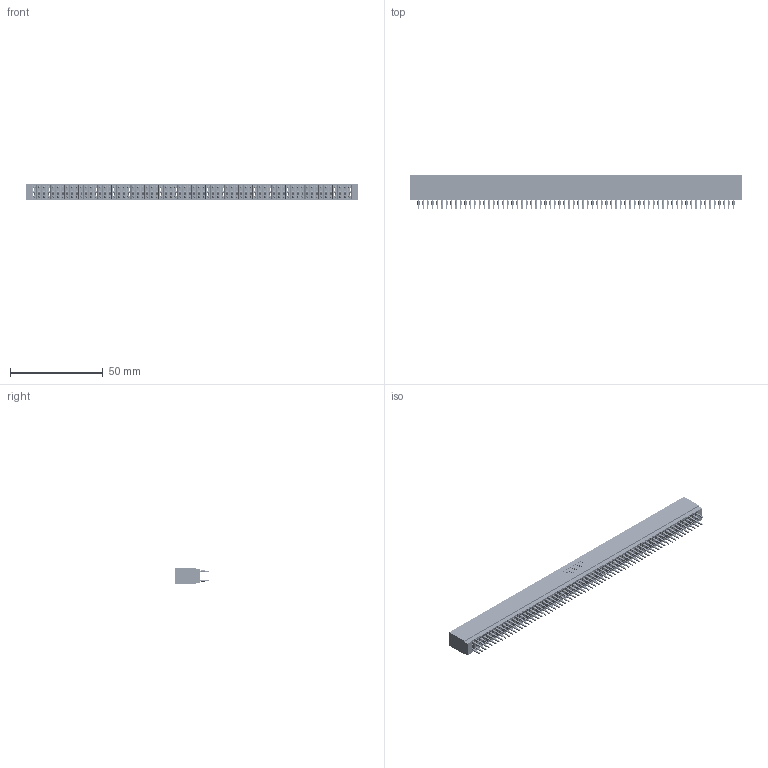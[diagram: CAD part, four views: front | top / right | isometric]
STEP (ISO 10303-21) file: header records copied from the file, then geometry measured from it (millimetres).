
FILE_DESCRIPTION (( 'STEP AP203' ), '1' );
FILE_NAME ('725-136-560-201.STEP', '2026-02-25T21:32:34', ( '' ), ( '' ), 'SwSTEP 2.0', 'SolidWorks 2023', '' );
FILE_SCHEMA (( 'CONFIG_CONTROL_DESIGN' ));
Length unit declared in the file: millimetre
Products named in the file (3): 745-292-001_560; 725-136-560-201; 725 Part_Insulator Option - 01
Assembly tree (137 placements, depth 2):
  725-136-560-201
    725 Part_Insulator Option - 01
    745-292-001_560  x136
Bounding box: 179.32 x 18.8 x 8.89 mm (x, y, z)
Volume: 14592 mm3; surface area: 33520.6 mm2
Topology: 137 solids, 137 shells, 13491 faces, 36906 edges, 23424 vertices
Faces by surface type: plane 6991, cylinder 2964, bspline 2720, torus 816
Entity records: 111217 total; most frequent: CARTESIAN_POINT 19785, ORIENTED_EDGE 19272, DIRECTION 16820, EDGE_CURVE 9636, VECTOR 9038, LINE 9038, VERTEX_POINT 6144, AXIS2_PLACEMENT_3D 3891
